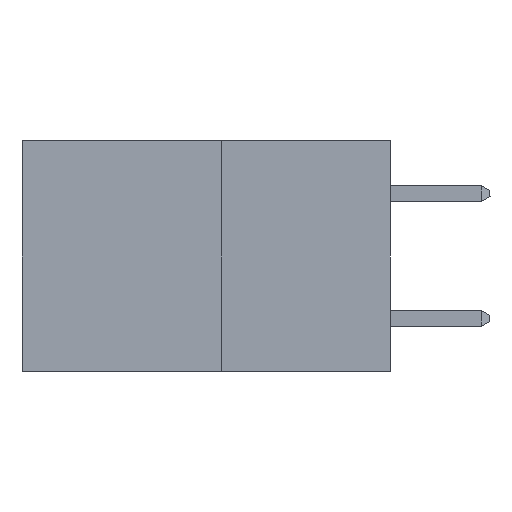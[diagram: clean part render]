
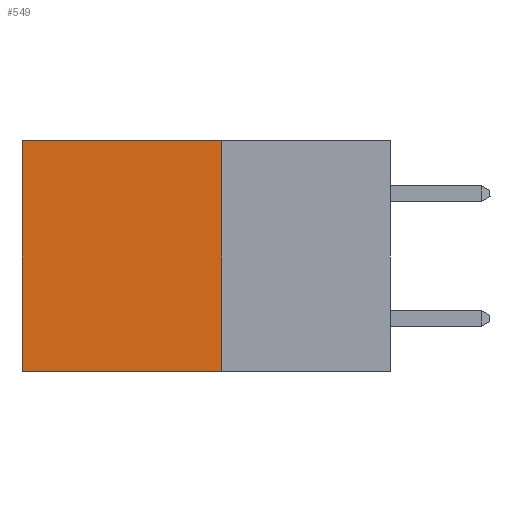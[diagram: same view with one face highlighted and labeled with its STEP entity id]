
A CAD part, left-side view. The second image highlights one B-rep face of the part: STEP entity #549.
In plain terms, the highlighted planar face has unit normal (-1, 0, 0).
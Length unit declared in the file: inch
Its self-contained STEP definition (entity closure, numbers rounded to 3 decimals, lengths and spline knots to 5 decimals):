
#549 = ADVANCED_FACE ( 'NONE', ( #2652 ), #29394, .F. ) ;
#2127 = ORIENTED_EDGE ( 'NONE', *, *, #26692, .F. ) ;
#2260 = DIRECTION ( 'NONE',  ( 0., 1., 0. ) ) ;
#2652 = FACE_OUTER_BOUND ( 'NONE', #23462, .T. ) ;
#4715 = CARTESIAN_POINT ( 'NONE',  ( 0.277, 0.59, -0.37 ) ) ;
#5152 = ORIENTED_EDGE ( 'NONE', *, *, #7212, .T. ) ;
#5243 = VECTOR ( 'NONE', #12044, 39.37008 ) ;
#7212 = EDGE_CURVE ( 'NONE', #29314, #9552, #27982, .T. ) ;
#8981 = AXIS2_PLACEMENT_3D ( 'NONE', #24761, #14188, #13758 ) ;
#9552 = VERTEX_POINT ( 'NONE', #29509 ) ;
#10734 = EDGE_CURVE ( 'NONE', #9552, #18559, #30805, .T. ) ;
#11038 = DIRECTION ( 'NONE',  ( 0., 1., 0. ) ) ;
#11537 = LINE ( 'NONE', #25404, #12310 ) ;
#12044 = DIRECTION ( 'NONE',  ( 0., 0., -1. ) ) ;
#12310 = VECTOR ( 'NONE', #11038, 39.37008 ) ;
#13758 = DIRECTION ( 'NONE',  ( 0., 0., -1. ) ) ;
#14188 = DIRECTION ( 'NONE',  ( 1., 0., 0. ) ) ;
#14322 = VERTEX_POINT ( 'NONE', #27790 ) ;
#14347 = CARTESIAN_POINT ( 'NONE',  ( 0.277, 0.27, 0. ) ) ;
#14502 = VECTOR ( 'NONE', #2260, 39.37008 ) ;
#15039 = CARTESIAN_POINT ( 'NONE',  ( 0.277, 0.27, -0.37 ) ) ;
#15277 = CARTESIAN_POINT ( 'NONE',  ( 0.277, 0.59, -0.37 ) ) ;
#16065 = ORIENTED_EDGE ( 'NONE', *, *, #27113, .F. ) ;
#17461 = DIRECTION ( 'NONE',  ( 0., 0., -1. ) ) ;
#17613 = VECTOR ( 'NONE', #17461, 39.37008 ) ;
#18355 = LINE ( 'NONE', #15039, #17613 ) ;
#18559 = VERTEX_POINT ( 'NONE', #15277 ) ;
#20240 = ORIENTED_EDGE ( 'NONE', *, *, #10734, .T. ) ;
#23462 = EDGE_LOOP ( 'NONE', ( #20240, #2127, #16065, #5152 ) ) ;
#24761 = CARTESIAN_POINT ( 'NONE',  ( 0.277, 0.27, -0.37 ) ) ;
#25404 = CARTESIAN_POINT ( 'NONE',  ( 0.277, 0.27, -0.37 ) ) ;
#26692 = EDGE_CURVE ( 'NONE', #14322, #18559, #11537, .T. ) ;
#27113 = EDGE_CURVE ( 'NONE', #29314, #14322, #18355, .T. ) ;
#27790 = CARTESIAN_POINT ( 'NONE',  ( 0.277, 0.27, -0.37 ) ) ;
#27982 = LINE ( 'NONE', #14347, #14502 ) ;
#29314 = VERTEX_POINT ( 'NONE', #29374 ) ;
#29374 = CARTESIAN_POINT ( 'NONE',  ( 0.277, 0.27, 0. ) ) ;
#29394 = PLANE ( 'NONE',  #8981 ) ;
#29509 = CARTESIAN_POINT ( 'NONE',  ( 0.277, 0.59, 0. ) ) ;
#30805 = LINE ( 'NONE', #4715, #5243 ) ;
